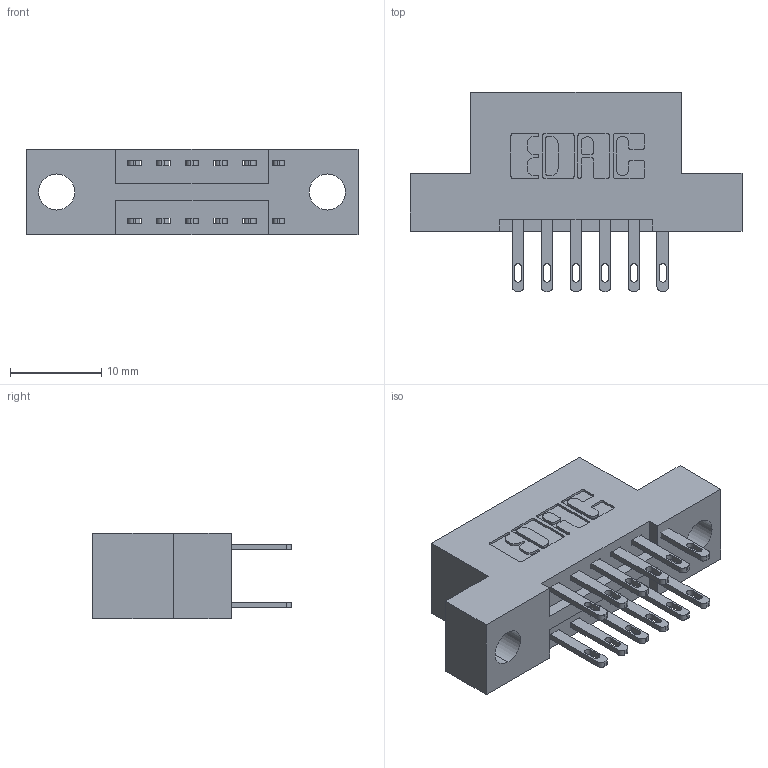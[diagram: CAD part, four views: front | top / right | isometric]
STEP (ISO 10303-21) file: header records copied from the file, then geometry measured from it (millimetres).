
FILE_DESCRIPTION (( 'STEP AP203' ), '1' );
FILE_NAME ('346-012-500-204.STEP', '2022-05-17T18:49:09', ( '' ), ( '' ), 'SwSTEP 2.0', 'SolidWorks 2020', '' );
FILE_SCHEMA (( 'CONFIG_CONTROL_DESIGN' ));
Length unit declared in the file: inch
Products named in the file (3): 345-292-001_345-293-100; 346-012-500-204; 346 Part_Flush Mounting Lugs - 0.156 Dia-TH
Assembly tree (13 placements, depth 2):
  346-012-500-204
    346 Part_Flush Mounting Lugs - 0.156 Dia-TH
    345-292-001_345-293-100  x12
Bounding box: 36.45 x 21.84 x 9.4 mm (x, y, z)
Volume: 3215.6 mm3; surface area: 3915.8 mm2
Topology: 13 solids, 13 shells, 700 faces, 2087 edges, 1390 vertices
Faces by surface type: plane 428, cylinder 272
Entity records: 8657 total; most frequent: CARTESIAN_POINT 1472, ORIENTED_EDGE 1402, DIRECTION 1353, EDGE_CURVE 701, VECTOR 545, LINE 545, VERTEX_POINT 466, AXIS2_PLACEMENT_3D 404
